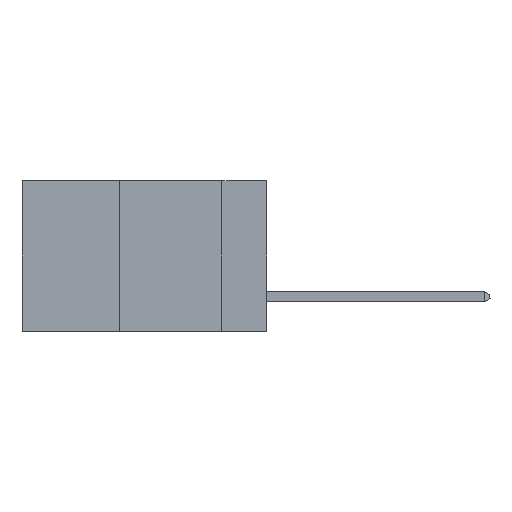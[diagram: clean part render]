
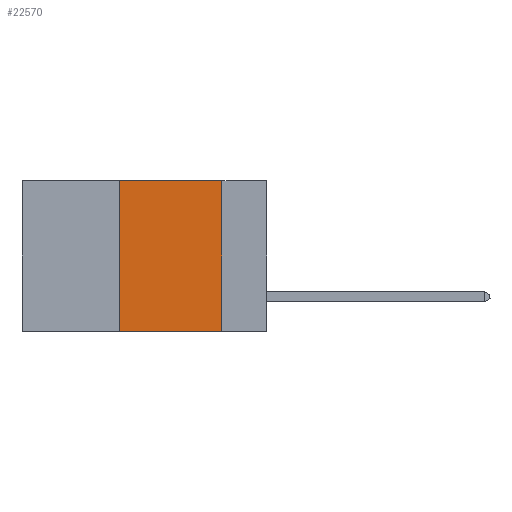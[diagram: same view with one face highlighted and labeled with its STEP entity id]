
A CAD part, left-side view. The second image highlights one B-rep face of the part: STEP entity #22570.
In plain terms, the highlighted planar face has unit normal (-1, 0, 0).
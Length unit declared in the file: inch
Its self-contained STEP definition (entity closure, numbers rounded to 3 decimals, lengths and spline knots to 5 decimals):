
#1432 = DIRECTION ( 'NONE',  ( 0., 0., 1. ) ) ;
#2922 = CARTESIAN_POINT ( 'NONE',  ( 0., 0.6, -0.37 ) ) ;
#3467 = VECTOR ( 'NONE', #20073, 39.37008 ) ;
#4699 = DIRECTION ( 'NONE',  ( 0., -1., 0. ) ) ;
#5574 = VECTOR ( 'NONE', #4699, 39.37008 ) ;
#7841 = VERTEX_POINT ( 'NONE', #10572 ) ;
#8822 = LINE ( 'NONE', #22007, #3467 ) ;
#10572 = CARTESIAN_POINT ( 'NONE',  ( 0., 0.11, -0.37 ) ) ;
#11058 = DIRECTION ( 'NONE',  ( 0., 0., -1. ) ) ;
#11243 = VERTEX_POINT ( 'NONE', #25684 ) ;
#11670 = VECTOR ( 'NONE', #22652, 39.37008 ) ;
#12326 = EDGE_CURVE ( 'NONE', #21912, #7841, #15349, .T. ) ;
#12439 = FACE_OUTER_BOUND ( 'NONE', #13843, .T. ) ;
#13010 = CARTESIAN_POINT ( 'NONE',  ( 0., 0.36, -0.37 ) ) ;
#13539 = LINE ( 'NONE', #22559, #11670 ) ;
#13843 = EDGE_LOOP ( 'NONE', ( #24403, #17897, #16712, #22143 ) ) ;
#15349 = LINE ( 'NONE', #2922, #5574 ) ;
#16204 = EDGE_CURVE ( 'NONE', #11243, #7841, #8822, .T. ) ;
#16457 = VECTOR ( 'NONE', #1432, 39.37008 ) ;
#16712 = ORIENTED_EDGE ( 'NONE', *, *, #18994, .F. ) ;
#17677 = AXIS2_PLACEMENT_3D ( 'NONE', #20635, #23285, #11058 ) ;
#17897 = ORIENTED_EDGE ( 'NONE', *, *, #25577, .F. ) ;
#18994 = EDGE_CURVE ( 'NONE', #21912, #19305, #22139, .T. ) ;
#19305 = VERTEX_POINT ( 'NONE', #22692 ) ;
#19518 = CARTESIAN_POINT ( 'NONE',  ( 0., 0.36, 0. ) ) ;
#20073 = DIRECTION ( 'NONE',  ( 0., 0., -1. ) ) ;
#20547 = PLANE ( 'NONE',  #17677 ) ;
#20635 = CARTESIAN_POINT ( 'NONE',  ( 0., 0.6, 0. ) ) ;
#21912 = VERTEX_POINT ( 'NONE', #13010 ) ;
#22007 = CARTESIAN_POINT ( 'NONE',  ( 0., 0.11, 0. ) ) ;
#22139 = LINE ( 'NONE', #19518, #16457 ) ;
#22143 = ORIENTED_EDGE ( 'NONE', *, *, #12326, .T. ) ;
#22559 = CARTESIAN_POINT ( 'NONE',  ( 0., 0.6, 0. ) ) ;
#22570 = ADVANCED_FACE ( 'NONE', ( #12439 ), #20547, .F. ) ;
#22652 = DIRECTION ( 'NONE',  ( 0., -1., 0. ) ) ;
#22692 = CARTESIAN_POINT ( 'NONE',  ( 0., 0.36, 0. ) ) ;
#23285 = DIRECTION ( 'NONE',  ( 1., 0., 0. ) ) ;
#24403 = ORIENTED_EDGE ( 'NONE', *, *, #16204, .F. ) ;
#25577 = EDGE_CURVE ( 'NONE', #19305, #11243, #13539, .T. ) ;
#25684 = CARTESIAN_POINT ( 'NONE',  ( 0., 0.11, 0. ) ) ;
